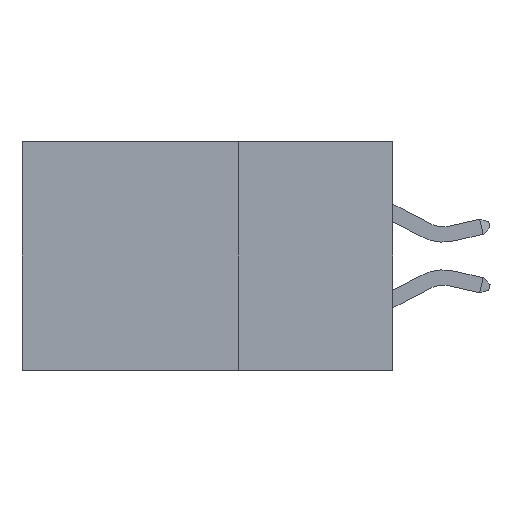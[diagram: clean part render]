
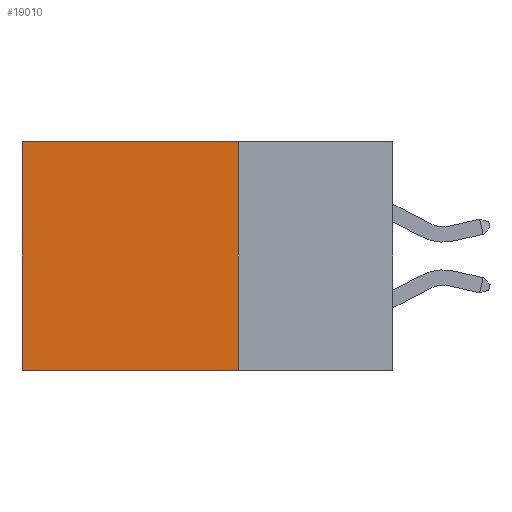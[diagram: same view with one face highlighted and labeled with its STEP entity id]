
A CAD part, left-side view. The second image highlights one B-rep face of the part: STEP entity #19010.
In plain terms, the highlighted planar face has unit normal (-1, 0, 0).
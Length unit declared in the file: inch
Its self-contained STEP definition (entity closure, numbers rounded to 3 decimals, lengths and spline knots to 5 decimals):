
#646 = LINE ( 'NONE', #9835, #7459 ) ;
#1054 = LINE ( 'NONE', #7746, #14432 ) ;
#1127 = ORIENTED_EDGE ( 'NONE', *, *, #19292, .T. ) ;
#3901 = CARTESIAN_POINT ( 'NONE',  ( 0.2875, 0.25, 0. ) ) ;
#4553 = VERTEX_POINT ( 'NONE', #15572 ) ;
#5001 = CARTESIAN_POINT ( 'NONE',  ( 0.2875, 0.25, 0. ) ) ;
#5747 = VECTOR ( 'NONE', #11938, 39.37008 ) ;
#5977 = EDGE_CURVE ( 'NONE', #15097, #22547, #1054, .T. ) ;
#6193 = ORIENTED_EDGE ( 'NONE', *, *, #16313, .F. ) ;
#6767 = ORIENTED_EDGE ( 'NONE', *, *, #12254, .T. ) ;
#7052 = LINE ( 'NONE', #19316, #18271 ) ;
#7099 = LINE ( 'NONE', #18587, #5747 ) ;
#7459 = VECTOR ( 'NONE', #13146, 39.37008 ) ;
#7746 = CARTESIAN_POINT ( 'NONE',  ( 0.2875, 0.25, 0. ) ) ;
#8577 = PLANE ( 'NONE',  #15474 ) ;
#9835 = CARTESIAN_POINT ( 'NONE',  ( 0.2875, 0.25, 0. ) ) ;
#10328 = DIRECTION ( 'NONE',  ( 0., 1., 0. ) ) ;
#10506 = CARTESIAN_POINT ( 'NONE',  ( 0.2875, 0.6, 0. ) ) ;
#11938 = DIRECTION ( 'NONE',  ( 0., 0., -1. ) ) ;
#12254 = EDGE_CURVE ( 'NONE', #15097, #21263, #646, .T. ) ;
#13146 = DIRECTION ( 'NONE',  ( 0., 1., 0. ) ) ;
#14432 = VECTOR ( 'NONE', #22013, 39.37008 ) ;
#14534 = ORIENTED_EDGE ( 'NONE', *, *, #5977, .F. ) ;
#15097 = VERTEX_POINT ( 'NONE', #3901 ) ;
#15474 = AXIS2_PLACEMENT_3D ( 'NONE', #5001, #15617, #19085 ) ;
#15572 = CARTESIAN_POINT ( 'NONE',  ( 0.2875, 0.6, -0.37 ) ) ;
#15617 = DIRECTION ( 'NONE',  ( 1., 0., 0. ) ) ;
#15740 = FACE_OUTER_BOUND ( 'NONE', #17886, .T. ) ;
#15829 = CARTESIAN_POINT ( 'NONE',  ( 0.2875, 0.25, -0.37 ) ) ;
#16313 = EDGE_CURVE ( 'NONE', #22547, #4553, #7052, .T. ) ;
#17886 = EDGE_LOOP ( 'NONE', ( #1127, #6193, #14534, #6767 ) ) ;
#18271 = VECTOR ( 'NONE', #10328, 39.37008 ) ;
#18587 = CARTESIAN_POINT ( 'NONE',  ( 0.2875, 0.6, 0. ) ) ;
#19010 = ADVANCED_FACE ( 'NONE', ( #15740 ), #8577, .F. ) ;
#19085 = DIRECTION ( 'NONE',  ( 0., 0., -1. ) ) ;
#19292 = EDGE_CURVE ( 'NONE', #21263, #4553, #7099, .T. ) ;
#19316 = CARTESIAN_POINT ( 'NONE',  ( 0.2875, 0.25, -0.37 ) ) ;
#21263 = VERTEX_POINT ( 'NONE', #10506 ) ;
#22013 = DIRECTION ( 'NONE',  ( 0., 0., -1. ) ) ;
#22547 = VERTEX_POINT ( 'NONE', #15829 ) ;
